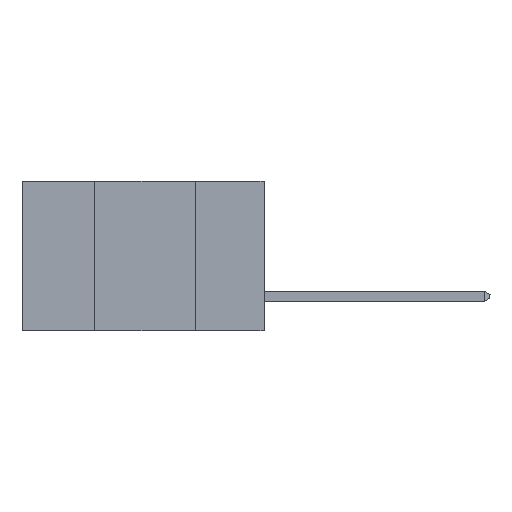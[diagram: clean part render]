
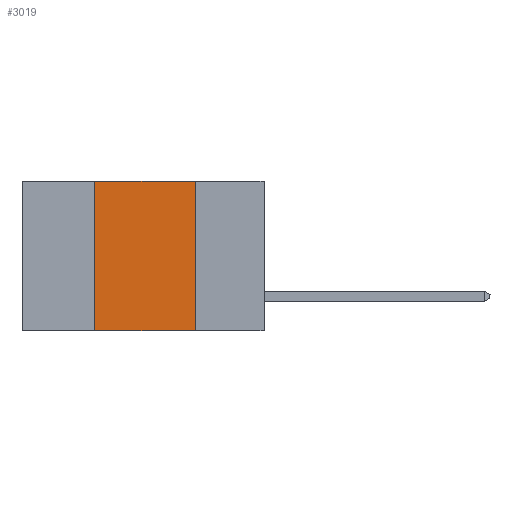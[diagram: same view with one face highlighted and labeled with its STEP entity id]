
A CAD part, left-side view. The second image highlights one B-rep face of the part: STEP entity #3019.
In plain terms, the highlighted planar face has unit normal (-1, 0, 0).
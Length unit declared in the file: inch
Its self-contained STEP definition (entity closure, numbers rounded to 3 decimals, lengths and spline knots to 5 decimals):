
#427 = CARTESIAN_POINT ( 'NONE',  ( 0., 0.17, 0. ) ) ;
#817 = ORIENTED_EDGE ( 'NONE', *, *, #5074, .F. ) ;
#2532 = FACE_OUTER_BOUND ( 'NONE', #8239, .T. ) ;
#3019 = ADVANCED_FACE ( 'NONE', ( #2532 ), #9513, .F. ) ;
#3043 = LINE ( 'NONE', #12767, #16311 ) ;
#3629 = LINE ( 'NONE', #11613, #13486 ) ;
#4069 = ORIENTED_EDGE ( 'NONE', *, *, #7637, .T. ) ;
#4468 = VERTEX_POINT ( 'NONE', #16455 ) ;
#4660 = CARTESIAN_POINT ( 'NONE',  ( 0., 0.42, -0.37 ) ) ;
#5074 = EDGE_CURVE ( 'NONE', #14322, #4468, #3043, .T. ) ;
#5286 = EDGE_CURVE ( 'NONE', #4468, #7991, #3629, .T. ) ;
#5588 = ORIENTED_EDGE ( 'NONE', *, *, #5286, .F. ) ;
#5713 = CARTESIAN_POINT ( 'NONE',  ( 0., 0.17, 0. ) ) ;
#5770 = CARTESIAN_POINT ( 'NONE',  ( 0., 0.6, 0. ) ) ;
#7637 = EDGE_CURVE ( 'NONE', #14322, #11961, #11715, .T. ) ;
#7991 = VERTEX_POINT ( 'NONE', #5713 ) ;
#8239 = EDGE_LOOP ( 'NONE', ( #14175, #5588, #817, #4069 ) ) ;
#9513 = PLANE ( 'NONE',  #11102 ) ;
#9638 = CARTESIAN_POINT ( 'NONE',  ( 0., 0.17, -0.37 ) ) ;
#10238 = DIRECTION ( 'NONE',  ( 0., 0., 1. ) ) ;
#10914 = VECTOR ( 'NONE', #13157, 39.37008 ) ;
#11102 = AXIS2_PLACEMENT_3D ( 'NONE', #5770, #13404, #12118 ) ;
#11613 = CARTESIAN_POINT ( 'NONE',  ( 0., 0.6, 0. ) ) ;
#11715 = LINE ( 'NONE', #14343, #10914 ) ;
#11961 = VERTEX_POINT ( 'NONE', #9638 ) ;
#12118 = DIRECTION ( 'NONE',  ( 0., 0., -1. ) ) ;
#12611 = EDGE_CURVE ( 'NONE', #7991, #11961, #14626, .T. ) ;
#12767 = CARTESIAN_POINT ( 'NONE',  ( 0., 0.42, 0. ) ) ;
#13157 = DIRECTION ( 'NONE',  ( 0., -1., 0. ) ) ;
#13323 = DIRECTION ( 'NONE',  ( 0., 0., -1. ) ) ;
#13404 = DIRECTION ( 'NONE',  ( 1., 0., 0. ) ) ;
#13416 = VECTOR ( 'NONE', #13323, 39.37008 ) ;
#13486 = VECTOR ( 'NONE', #14306, 39.37008 ) ;
#14175 = ORIENTED_EDGE ( 'NONE', *, *, #12611, .F. ) ;
#14306 = DIRECTION ( 'NONE',  ( 0., -1., 0. ) ) ;
#14322 = VERTEX_POINT ( 'NONE', #4660 ) ;
#14343 = CARTESIAN_POINT ( 'NONE',  ( 0., 0.6, -0.37 ) ) ;
#14626 = LINE ( 'NONE', #427, #13416 ) ;
#16311 = VECTOR ( 'NONE', #10238, 39.37008 ) ;
#16455 = CARTESIAN_POINT ( 'NONE',  ( 0., 0.42, 0. ) ) ;
